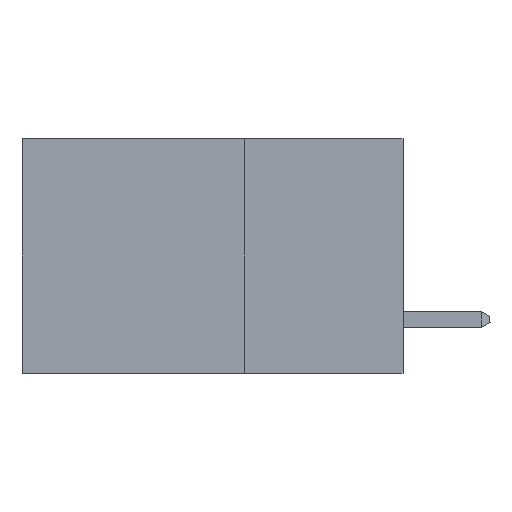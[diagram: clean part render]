
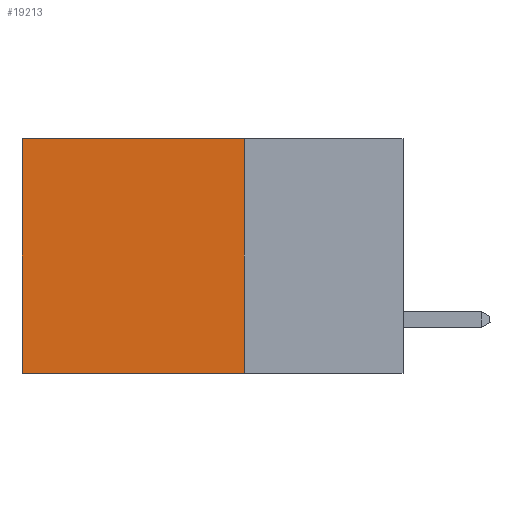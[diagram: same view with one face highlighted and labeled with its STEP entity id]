
A CAD part, left-side view. The second image highlights one B-rep face of the part: STEP entity #19213.
In plain terms, the highlighted planar face has unit normal (-1, 0, 0).
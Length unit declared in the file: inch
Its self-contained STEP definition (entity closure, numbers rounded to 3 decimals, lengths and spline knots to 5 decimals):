
#308 = LINE ( 'NONE', #6930, #23697 ) ;
#381 = ORIENTED_EDGE ( 'NONE', *, *, #24310, .F. ) ;
#388 = VECTOR ( 'NONE', #14549, 39.37008 ) ;
#934 = CARTESIAN_POINT ( 'NONE',  ( 0.2875, 0.25, -0.37 ) ) ;
#3212 = FACE_OUTER_BOUND ( 'NONE', #5553, .T. ) ;
#5185 = EDGE_CURVE ( 'NONE', #41900, #6144, #9527, .T. ) ;
#5553 = EDGE_LOOP ( 'NONE', ( #20909, #24594, #381, #37595 ) ) ;
#6144 = VERTEX_POINT ( 'NONE', #26762 ) ;
#6930 = CARTESIAN_POINT ( 'NONE',  ( 0.2875, 0.25, 0. ) ) ;
#9527 = LINE ( 'NONE', #20818, #23319 ) ;
#11734 = CARTESIAN_POINT ( 'NONE',  ( 0.2875, 0.6, 0. ) ) ;
#13636 = CARTESIAN_POINT ( 'NONE',  ( 0.2875, 0.25, 0. ) ) ;
#14130 = EDGE_CURVE ( 'NONE', #32899, #16722, #16397, .T. ) ;
#14549 = DIRECTION ( 'NONE',  ( 0., 0., -1. ) ) ;
#16397 = LINE ( 'NONE', #41958, #28675 ) ;
#16722 = VERTEX_POINT ( 'NONE', #30005 ) ;
#19213 = ADVANCED_FACE ( 'NONE', ( #3212 ), #43394, .F. ) ;
#20818 = CARTESIAN_POINT ( 'NONE',  ( 0.2875, 0.25, 0. ) ) ;
#20909 = ORIENTED_EDGE ( 'NONE', *, *, #23496, .T. ) ;
#23319 = VECTOR ( 'NONE', #27872, 39.37008 ) ;
#23496 = EDGE_CURVE ( 'NONE', #6144, #16722, #41351, .T. ) ;
#23697 = VECTOR ( 'NONE', #41438, 39.37008 ) ;
#24310 = EDGE_CURVE ( 'NONE', #41900, #32899, #308, .T. ) ;
#24594 = ORIENTED_EDGE ( 'NONE', *, *, #14130, .F. ) ;
#26762 = CARTESIAN_POINT ( 'NONE',  ( 0.2875, 0.6, 0. ) ) ;
#27872 = DIRECTION ( 'NONE',  ( 0., 1., 0. ) ) ;
#28675 = VECTOR ( 'NONE', #31826, 39.37008 ) ;
#28682 = AXIS2_PLACEMENT_3D ( 'NONE', #13636, #40878, #37718 ) ;
#30005 = CARTESIAN_POINT ( 'NONE',  ( 0.2875, 0.6, -0.37 ) ) ;
#31826 = DIRECTION ( 'NONE',  ( 0., 1., 0. ) ) ;
#32899 = VERTEX_POINT ( 'NONE', #934 ) ;
#36556 = CARTESIAN_POINT ( 'NONE',  ( 0.2875, 0.25, 0. ) ) ;
#37595 = ORIENTED_EDGE ( 'NONE', *, *, #5185, .T. ) ;
#37718 = DIRECTION ( 'NONE',  ( 0., 0., -1. ) ) ;
#40878 = DIRECTION ( 'NONE',  ( 1., 0., 0. ) ) ;
#41351 = LINE ( 'NONE', #11734, #388 ) ;
#41438 = DIRECTION ( 'NONE',  ( 0., 0., -1. ) ) ;
#41900 = VERTEX_POINT ( 'NONE', #36556 ) ;
#41958 = CARTESIAN_POINT ( 'NONE',  ( 0.2875, 0.25, -0.37 ) ) ;
#43394 = PLANE ( 'NONE',  #28682 ) ;
